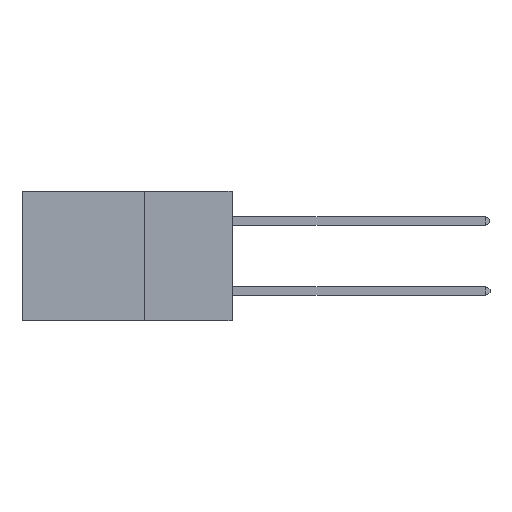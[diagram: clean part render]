
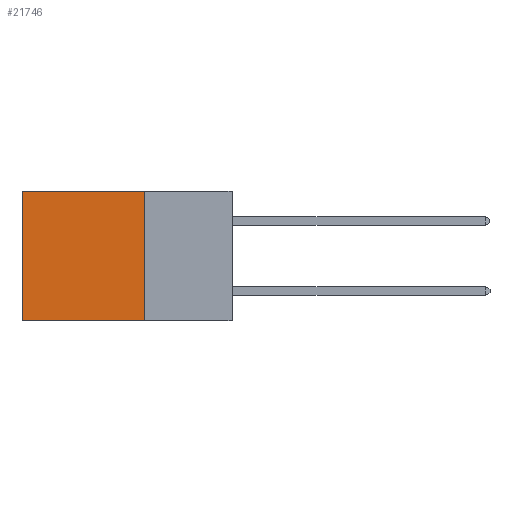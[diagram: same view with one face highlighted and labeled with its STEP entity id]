
A CAD part, left-side view. The second image highlights one B-rep face of the part: STEP entity #21746.
In plain terms, the highlighted planar face has unit normal (-1, 0, 0).
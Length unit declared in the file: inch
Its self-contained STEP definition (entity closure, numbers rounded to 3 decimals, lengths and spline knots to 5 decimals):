
#377 = ORIENTED_EDGE ( 'NONE', *, *, #4722, .T. ) ;
#3966 = VERTEX_POINT ( 'NONE', #6572 ) ;
#4342 = DIRECTION ( 'NONE',  ( 1., 0., 0. ) ) ;
#4722 = EDGE_CURVE ( 'NONE', #23029, #19748, #12598, .T. ) ;
#4982 = DIRECTION ( 'NONE',  ( 0., 0., -1. ) ) ;
#5265 = ORIENTED_EDGE ( 'NONE', *, *, #17347, .F. ) ;
#5842 = DIRECTION ( 'NONE',  ( 0., 0., -1. ) ) ;
#6572 = CARTESIAN_POINT ( 'NONE',  ( 0.2875, 0.25, -0.37 ) ) ;
#6996 = FACE_OUTER_BOUND ( 'NONE', #10776, .T. ) ;
#7830 = DIRECTION ( 'NONE',  ( 0., 1., 0. ) ) ;
#8440 = VECTOR ( 'NONE', #17866, 39.37008 ) ;
#8619 = EDGE_CURVE ( 'NONE', #23029, #3966, #9634, .T. ) ;
#8772 = AXIS2_PLACEMENT_3D ( 'NONE', #11402, #4342, #5842 ) ;
#8817 = CARTESIAN_POINT ( 'NONE',  ( 0.2875, 0.6, 0. ) ) ;
#9248 = EDGE_CURVE ( 'NONE', #19748, #15821, #16425, .T. ) ;
#9457 = PLANE ( 'NONE',  #8772 ) ;
#9634 = LINE ( 'NONE', #13440, #19957 ) ;
#10776 = EDGE_LOOP ( 'NONE', ( #22733, #5265, #12221, #377 ) ) ;
#11402 = CARTESIAN_POINT ( 'NONE',  ( 0.2875, 0.25, 0. ) ) ;
#11502 = DIRECTION ( 'NONE',  ( 0., 0., -1. ) ) ;
#12221 = ORIENTED_EDGE ( 'NONE', *, *, #8619, .F. ) ;
#12598 = LINE ( 'NONE', #21261, #23547 ) ;
#12633 = CARTESIAN_POINT ( 'NONE',  ( 0.2875, 0.6, 0. ) ) ;
#13440 = CARTESIAN_POINT ( 'NONE',  ( 0.2875, 0.25, 0. ) ) ;
#13577 = CARTESIAN_POINT ( 'NONE',  ( 0.2875, 0.6, -0.37 ) ) ;
#15821 = VERTEX_POINT ( 'NONE', #13577 ) ;
#16425 = LINE ( 'NONE', #12633, #20984 ) ;
#17347 = EDGE_CURVE ( 'NONE', #3966, #15821, #19636, .T. ) ;
#17539 = CARTESIAN_POINT ( 'NONE',  ( 0.2875, 0.25, 0. ) ) ;
#17866 = DIRECTION ( 'NONE',  ( 0., 1., 0. ) ) ;
#19636 = LINE ( 'NONE', #21855, #8440 ) ;
#19748 = VERTEX_POINT ( 'NONE', #8817 ) ;
#19957 = VECTOR ( 'NONE', #11502, 39.37008 ) ;
#20984 = VECTOR ( 'NONE', #4982, 39.37008 ) ;
#21261 = CARTESIAN_POINT ( 'NONE',  ( 0.2875, 0.25, 0. ) ) ;
#21746 = ADVANCED_FACE ( 'NONE', ( #6996 ), #9457, .F. ) ;
#21855 = CARTESIAN_POINT ( 'NONE',  ( 0.2875, 0.25, -0.37 ) ) ;
#22733 = ORIENTED_EDGE ( 'NONE', *, *, #9248, .T. ) ;
#23029 = VERTEX_POINT ( 'NONE', #17539 ) ;
#23547 = VECTOR ( 'NONE', #7830, 39.37008 ) ;
